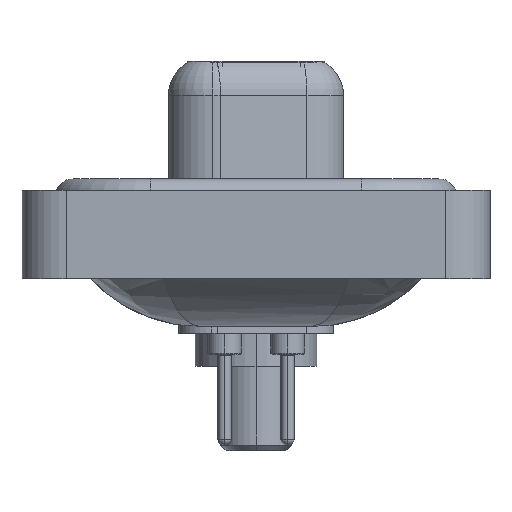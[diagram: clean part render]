
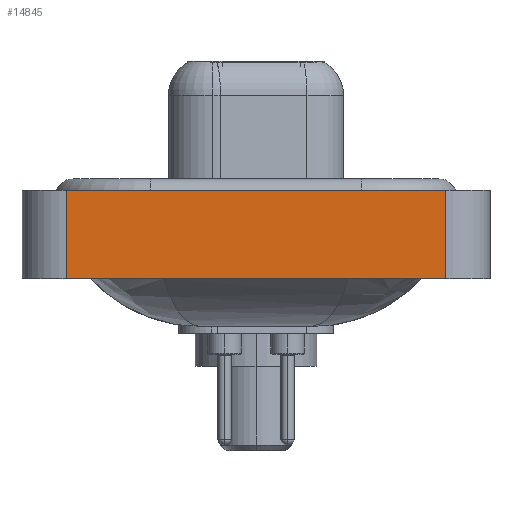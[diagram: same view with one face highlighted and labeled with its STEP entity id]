
A CAD part, left-side view. The second image highlights one B-rep face of the part: STEP entity #14845.
In plain terms, the highlighted planar face has unit normal (-1, 0, 0).
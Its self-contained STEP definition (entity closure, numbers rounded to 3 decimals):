
#121 = DIRECTION ( 'NONE',  ( 0., 0., 1. ) ) ;
#900 = DIRECTION ( 'NONE',  ( 0., -1., 0. ) ) ;
#2028 = VERTEX_POINT ( 'NONE', #4556 ) ;
#2996 = VECTOR ( 'NONE', #3509, 1000. ) ;
#3289 = CARTESIAN_POINT ( 'NONE',  ( -7.35, 8.55, 0.4 ) ) ;
#3509 = DIRECTION ( 'NONE',  ( 0., 0., 1. ) ) ;
#3553 = ORIENTED_EDGE ( 'NONE', *, *, #3768, .T. ) ;
#3768 = EDGE_CURVE ( 'NONE', #2028, #7220, #9049, .T. ) ;
#3933 = VECTOR ( 'NONE', #23132, 1000. ) ;
#4556 = CARTESIAN_POINT ( 'NONE',  ( -7.35, -8.55, -3.6 ) ) ;
#5928 = FACE_OUTER_BOUND ( 'NONE', #17409, .T. ) ;
#7220 = VERTEX_POINT ( 'NONE', #23374 ) ;
#9049 = LINE ( 'NONE', #25525, #2996 ) ;
#10276 = DIRECTION ( 'NONE',  ( 0., 0., 1. ) ) ;
#10397 = VERTEX_POINT ( 'NONE', #3289 ) ;
#10557 = VECTOR ( 'NONE', #10276, 1000. ) ;
#11259 = CARTESIAN_POINT ( 'NONE',  ( -7.35, -8.55, -3.6 ) ) ;
#13864 = EDGE_CURVE ( 'NONE', #18268, #10397, #23997, .T. ) ;
#14270 = ORIENTED_EDGE ( 'NONE', *, *, #13864, .F. ) ;
#14774 = CARTESIAN_POINT ( 'NONE',  ( -7.35, 8.55, -3.6 ) ) ;
#14845 = ADVANCED_FACE ( 'NONE', ( #5928 ), #16214, .T. ) ;
#15004 = CARTESIAN_POINT ( 'NONE',  ( -7.35, -8.55, 0.4 ) ) ;
#15550 = ORIENTED_EDGE ( 'NONE', *, *, #22788, .F. ) ;
#16214 = PLANE ( 'NONE',  #18984 ) ;
#17104 = LINE ( 'NONE', #15004, #18407 ) ;
#17409 = EDGE_LOOP ( 'NONE', ( #3553, #15550, #14270, #25271 ) ) ;
#17451 = LINE ( 'NONE', #11259, #3933 ) ;
#18268 = VERTEX_POINT ( 'NONE', #14774 ) ;
#18407 = VECTOR ( 'NONE', #900, 1000. ) ;
#18984 = AXIS2_PLACEMENT_3D ( 'NONE', #22039, #24525, #121 ) ;
#19803 = CARTESIAN_POINT ( 'NONE',  ( -7.35, 8.55, -3.6 ) ) ;
#22039 = CARTESIAN_POINT ( 'NONE',  ( -7.35, -8.55, -3.6 ) ) ;
#22788 = EDGE_CURVE ( 'NONE', #10397, #7220, #17104, .T. ) ;
#23132 = DIRECTION ( 'NONE',  ( 0., -1., 0. ) ) ;
#23374 = CARTESIAN_POINT ( 'NONE',  ( -7.35, -8.55, 0.4 ) ) ;
#23997 = LINE ( 'NONE', #19803, #10557 ) ;
#24525 = DIRECTION ( 'NONE',  ( -1., 0., 0. ) ) ;
#24996 = EDGE_CURVE ( 'NONE', #18268, #2028, #17451, .T. ) ;
#25271 = ORIENTED_EDGE ( 'NONE', *, *, #24996, .T. ) ;
#25525 = CARTESIAN_POINT ( 'NONE',  ( -7.35, -8.55, -3.6 ) ) ;
